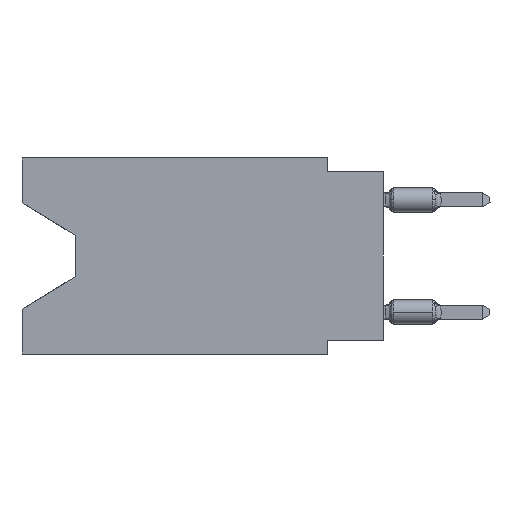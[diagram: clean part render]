
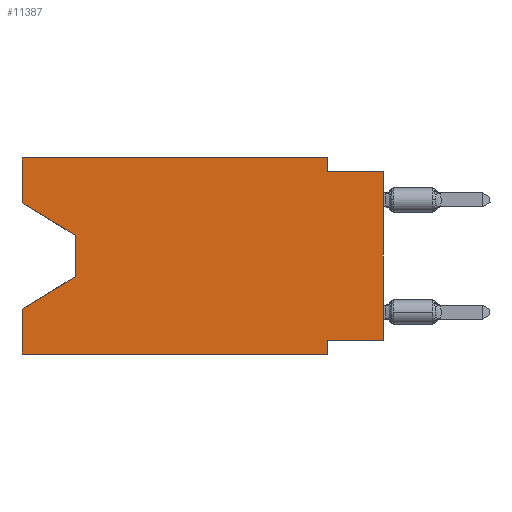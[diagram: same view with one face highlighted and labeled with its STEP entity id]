
A CAD part, left-side view. The second image highlights one B-rep face of the part: STEP entity #11387.
In plain terms, the highlighted planar face has unit normal (-1, 0, 0).
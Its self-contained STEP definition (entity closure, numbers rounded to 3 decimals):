
#202 = ORIENTED_EDGE ( 'NONE', *, *, #14129, .F. ) ;
#752 = VERTEX_POINT ( 'NONE', #25912 ) ;
#914 = ORIENTED_EDGE ( 'NONE', *, *, #31171, .F. ) ;
#1837 = CARTESIAN_POINT ( 'NONE',  ( 0., 16.383, -2.038 ) ) ;
#2105 = CARTESIAN_POINT ( 'NONE',  ( 0., 16.383, 0. ) ) ;
#2603 = EDGE_CURVE ( 'NONE', #24885, #14789, #6735, .T. ) ;
#3093 = VERTEX_POINT ( 'NONE', #20159 ) ;
#3236 = DIRECTION ( 'NONE',  ( 0., 0., -1. ) ) ;
#3729 = ORIENTED_EDGE ( 'NONE', *, *, #38572, .T. ) ;
#3888 = VECTOR ( 'NONE', #26431, 1000. ) ;
#4431 = DIRECTION ( 'NONE',  ( 0., -0.855, -0.519 ) ) ;
#5071 = ORIENTED_EDGE ( 'NONE', *, *, #11842, .F. ) ;
#6106 = VECTOR ( 'NONE', #9534, 1000. ) ;
#6735 = LINE ( 'NONE', #30366, #22969 ) ;
#6853 = EDGE_CURVE ( 'NONE', #31612, #752, #14722, .T. ) ;
#6861 = LINE ( 'NONE', #30881, #37069 ) ;
#6992 = CARTESIAN_POINT ( 'NONE',  ( 0., 16.383, -2.038 ) ) ;
#7521 = EDGE_CURVE ( 'NONE', #34423, #14789, #34905, .T. ) ;
#7591 = LINE ( 'NONE', #28461, #25196 ) ;
#9180 = CARTESIAN_POINT ( 'NONE',  ( 0., 16.383, 0. ) ) ;
#9500 = ORIENTED_EDGE ( 'NONE', *, *, #6853, .T. ) ;
#9534 = DIRECTION ( 'NONE',  ( 0., -1., 0. ) ) ;
#9556 = DIRECTION ( 'NONE',  ( 0., 0., -1. ) ) ;
#10702 = CARTESIAN_POINT ( 'NONE',  ( 0., 13.97, -5.385 ) ) ;
#11387 = ADVANCED_FACE ( 'NONE', ( #15096 ), #15675, .F. ) ;
#11842 = EDGE_CURVE ( 'NONE', #27009, #3093, #27253, .T. ) ;
#11847 = CARTESIAN_POINT ( 'NONE',  ( 0., 13.97, -3.505 ) ) ;
#11880 = VERTEX_POINT ( 'NONE', #37059 ) ;
#13895 = ORIENTED_EDGE ( 'NONE', *, *, #7521, .T. ) ;
#13992 = VECTOR ( 'NONE', #24860, 1000. ) ;
#14114 = DIRECTION ( 'NONE',  ( 0., 0., 1. ) ) ;
#14129 = EDGE_CURVE ( 'NONE', #29741, #37622, #20042, .T. ) ;
#14706 = VERTEX_POINT ( 'NONE', #37142 ) ;
#14722 = LINE ( 'NONE', #36534, #38700 ) ;
#14789 = VERTEX_POINT ( 'NONE', #23173 ) ;
#15096 = FACE_OUTER_BOUND ( 'NONE', #16895, .T. ) ;
#15337 = CARTESIAN_POINT ( 'NONE',  ( 0., 13.97, -5.385 ) ) ;
#15391 = DIRECTION ( 'NONE',  ( 0., 0., -1. ) ) ;
#15413 = VECTOR ( 'NONE', #4431, 1000. ) ;
#15675 = PLANE ( 'NONE',  #26667 ) ;
#16205 = EDGE_CURVE ( 'NONE', #31612, #27009, #16217, .T. ) ;
#16217 = LINE ( 'NONE', #18981, #13992 ) ;
#16447 = LINE ( 'NONE', #6992, #15413 ) ;
#16525 = CARTESIAN_POINT ( 'NONE',  ( 0., 16.383, 0. ) ) ;
#16602 = CARTESIAN_POINT ( 'NONE',  ( 0., 16.383, -8.89 ) ) ;
#16895 = EDGE_LOOP ( 'NONE', ( #36408, #32965, #13895, #35222, #3729, #5071, #37779, #9500, #30838, #914, #27647, #202 ) ) ;
#17801 = CARTESIAN_POINT ( 'NONE',  ( 0., 2.54, -8.255 ) ) ;
#17813 = CARTESIAN_POINT ( 'NONE',  ( 0., 2.54, -8.89 ) ) ;
#18981 = CARTESIAN_POINT ( 'NONE',  ( 0., 0., -8.255 ) ) ;
#19779 = VECTOR ( 'NONE', #15391, 1000. ) ;
#19972 = VECTOR ( 'NONE', #14114, 1000. ) ;
#20042 = LINE ( 'NONE', #2105, #19972 ) ;
#20159 = CARTESIAN_POINT ( 'NONE',  ( 0., 2.54, -8.89 ) ) ;
#21314 = DIRECTION ( 'NONE',  ( 0., 0., 1. ) ) ;
#22228 = VECTOR ( 'NONE', #30009, 1000. ) ;
#22969 = VECTOR ( 'NONE', #21314, 1000. ) ;
#23173 = CARTESIAN_POINT ( 'NONE',  ( 0., 16.383, -6.852 ) ) ;
#23665 = DIRECTION ( 'NONE',  ( 0., 0., -1. ) ) ;
#24201 = EDGE_CURVE ( 'NONE', #29741, #32477, #16447, .T. ) ;
#24541 = DIRECTION ( 'NONE',  ( 0., 0., 1. ) ) ;
#24860 = DIRECTION ( 'NONE',  ( 0., 1., 0. ) ) ;
#24885 = VERTEX_POINT ( 'NONE', #16602 ) ;
#25196 = VECTOR ( 'NONE', #23665, 1000. ) ;
#25717 = EDGE_CURVE ( 'NONE', #11880, #752, #27052, .T. ) ;
#25912 = CARTESIAN_POINT ( 'NONE',  ( 0., 0., -0.635 ) ) ;
#26185 = EDGE_CURVE ( 'NONE', #32477, #34423, #38808, .T. ) ;
#26431 = DIRECTION ( 'NONE',  ( 0., 0.855, -0.519 ) ) ;
#26667 = AXIS2_PLACEMENT_3D ( 'NONE', #9180, #29858, #9556 ) ;
#26884 = CARTESIAN_POINT ( 'NONE',  ( 0., 16.383, -8.89 ) ) ;
#27009 = VERTEX_POINT ( 'NONE', #17801 ) ;
#27052 = LINE ( 'NONE', #30202, #22228 ) ;
#27253 = LINE ( 'NONE', #17813, #36127 ) ;
#27354 = DIRECTION ( 'NONE',  ( 0., -1., 0. ) ) ;
#27647 = ORIENTED_EDGE ( 'NONE', *, *, #30408, .F. ) ;
#28461 = CARTESIAN_POINT ( 'NONE',  ( 0., 2.54, 0. ) ) ;
#29131 = CARTESIAN_POINT ( 'NONE',  ( 0., 0., -8.255 ) ) ;
#29622 = CARTESIAN_POINT ( 'NONE',  ( 0., 13.97, -3.505 ) ) ;
#29741 = VERTEX_POINT ( 'NONE', #1837 ) ;
#29858 = DIRECTION ( 'NONE',  ( 1., 0., 0. ) ) ;
#30009 = DIRECTION ( 'NONE',  ( 0., -1., 0. ) ) ;
#30202 = CARTESIAN_POINT ( 'NONE',  ( 0., 0., -0.635 ) ) ;
#30366 = CARTESIAN_POINT ( 'NONE',  ( 0., 16.383, 0. ) ) ;
#30408 = EDGE_CURVE ( 'NONE', #37622, #14706, #6861, .T. ) ;
#30838 = ORIENTED_EDGE ( 'NONE', *, *, #25717, .F. ) ;
#30881 = CARTESIAN_POINT ( 'NONE',  ( 0., 16.383, 0. ) ) ;
#31171 = EDGE_CURVE ( 'NONE', #14706, #11880, #7591, .T. ) ;
#31612 = VERTEX_POINT ( 'NONE', #29131 ) ;
#32477 = VERTEX_POINT ( 'NONE', #29622 ) ;
#32965 = ORIENTED_EDGE ( 'NONE', *, *, #26185, .T. ) ;
#34423 = VERTEX_POINT ( 'NONE', #15337 ) ;
#34905 = LINE ( 'NONE', #10702, #3888 ) ;
#35222 = ORIENTED_EDGE ( 'NONE', *, *, #2603, .F. ) ;
#35913 = LINE ( 'NONE', #26884, #6106 ) ;
#36127 = VECTOR ( 'NONE', #3236, 1000. ) ;
#36408 = ORIENTED_EDGE ( 'NONE', *, *, #24201, .T. ) ;
#36534 = CARTESIAN_POINT ( 'NONE',  ( 0., 0., 0. ) ) ;
#37059 = CARTESIAN_POINT ( 'NONE',  ( 0., 2.54, -0.635 ) ) ;
#37069 = VECTOR ( 'NONE', #27354, 1000. ) ;
#37142 = CARTESIAN_POINT ( 'NONE',  ( 0., 2.54, 0. ) ) ;
#37622 = VERTEX_POINT ( 'NONE', #16525 ) ;
#37779 = ORIENTED_EDGE ( 'NONE', *, *, #16205, .F. ) ;
#38572 = EDGE_CURVE ( 'NONE', #24885, #3093, #35913, .T. ) ;
#38700 = VECTOR ( 'NONE', #24541, 1000. ) ;
#38808 = LINE ( 'NONE', #11847, #19779 ) ;
